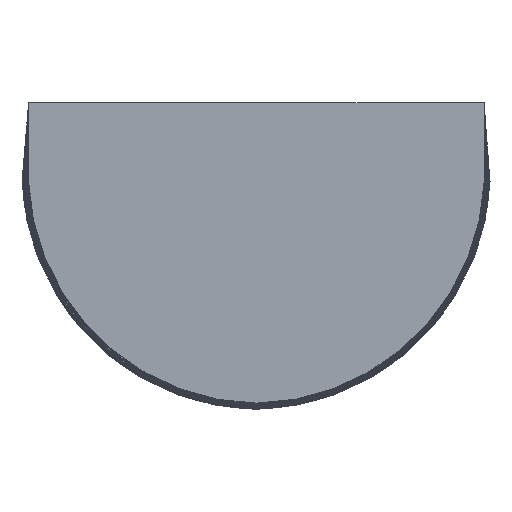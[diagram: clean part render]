
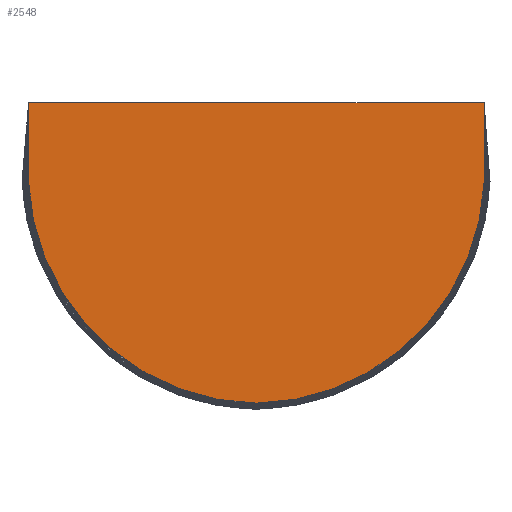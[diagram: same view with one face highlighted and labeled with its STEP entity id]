
A CAD part, front view. The second image highlights one B-rep face of the part: STEP entity #2548.
In plain terms, the highlighted planar face has unit normal (0, -1, 0).
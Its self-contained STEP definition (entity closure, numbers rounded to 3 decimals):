
#123=CIRCLE('',#2743,6.705);
#124=CIRCLE('',#2744,6.705);
#224=FACE_OUTER_BOUND('',#363,.T.);
#363=EDGE_LOOP('',(#1778,#1779,#1780,#1781,#1782));
#515=LINE('',#3567,#734);
#540=LINE('',#3662,#759);
#542=LINE('',#3666,#761);
#734=VECTOR('',#2947,10.);
#759=VECTOR('',#3016,10.);
#761=VECTOR('',#3020,10.);
#1051=VERTEX_POINT('',#3564);
#1052=VERTEX_POINT('',#3566);
#1094=VERTEX_POINT('',#3661);
#1095=VERTEX_POINT('',#3665);
#1096=VERTEX_POINT('',#3667);
#1320=EDGE_CURVE('',#1052,#1051,#515,.T.);
#1365=EDGE_CURVE('',#1094,#1052,#540,.T.);
#1367=EDGE_CURVE('',#1051,#1095,#542,.T.);
#1368=EDGE_CURVE('',#1095,#1096,#123,.T.);
#1369=EDGE_CURVE('',#1096,#1094,#124,.T.);
#1778=ORIENTED_EDGE('',*,*,#1320,.T.);
#1779=ORIENTED_EDGE('',*,*,#1367,.T.);
#1780=ORIENTED_EDGE('',*,*,#1368,.T.);
#1781=ORIENTED_EDGE('',*,*,#1369,.T.);
#1782=ORIENTED_EDGE('',*,*,#1365,.T.);
#2508=PLANE('',#2742);
#2548=ADVANCED_FACE('',(#224),#2508,.F.);
#2742=AXIS2_PLACEMENT_3D('',#3664,#3018,#3019);
#2743=AXIS2_PLACEMENT_3D('',#3668,#3021,#3022);
#2744=AXIS2_PLACEMENT_3D('',#3669,#3023,#3024);
#2947=DIRECTION('',(-1.,0.,0.));
#3016=DIRECTION('',(0.,0.,1.));
#3018=DIRECTION('center_axis',(0.,1.,0.));
#3019=DIRECTION('ref_axis',(0.,0.,1.));
#3020=DIRECTION('',(0.,0.,-1.));
#3021=DIRECTION('center_axis',(0.,-1.,0.));
#3022=DIRECTION('ref_axis',(-0.017,0.,-1.));
#3023=DIRECTION('center_axis',(0.,-1.,0.));
#3024=DIRECTION('ref_axis',(0.999,0.,-0.046));
#3564=CARTESIAN_POINT('',(-19.261,-239.951,-49.838));
#3566=CARTESIAN_POINT('',(-6.092,-239.95,-49.838));
#3567=CARTESIAN_POINT('',(-13.673,-239.95,-49.838));
#3661=CARTESIAN_POINT('',(-6.092,-239.95,-52.126));
#3662=CARTESIAN_POINT('',(-6.092,-239.95,-52.126));
#3664=CARTESIAN_POINT('Origin',(-12.677,-239.95,-39.838));
#3665=CARTESIAN_POINT('',(-19.261,-239.951,-52.126));
#3666=CARTESIAN_POINT('',(-19.261,-239.951,-27.55));
#3667=CARTESIAN_POINT('',(-12.677,-239.95,-58.524));
#3668=CARTESIAN_POINT('Origin',(-12.563,-239.95,-51.82));
#3669=CARTESIAN_POINT('Origin',(-12.79,-239.95,-51.82));
